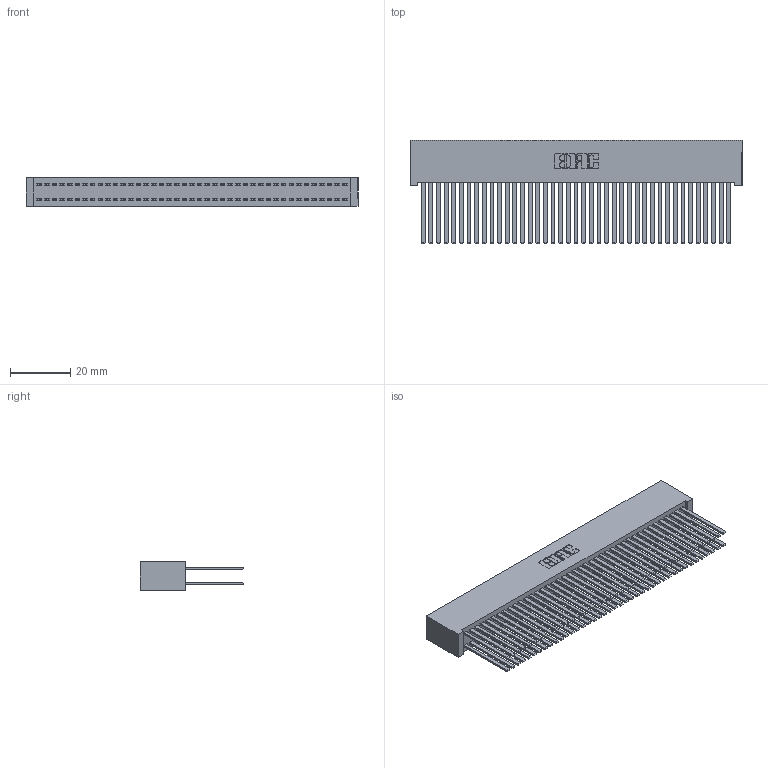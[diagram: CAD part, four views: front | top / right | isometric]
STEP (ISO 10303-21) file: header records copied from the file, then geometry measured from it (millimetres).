
FILE_DESCRIPTION (( 'STEP AP203' ), '1' );
FILE_NAME ('342-082-544-201.STEP', '2019-10-04T12:13:11', ( '' ), ( '' ), 'SwSTEP 2.0', 'SolidWorks 2016', '' );
FILE_SCHEMA (( 'CONFIG_CONTROL_DESIGN' ));
Length unit declared in the file: inch
Products named in the file (3): 342-082-544-201; 342 Part_Lugless; 345-292-001_345-293-144
Assembly tree (83 placements, depth 2):
  342-082-544-201
    342 Part_Lugless
    345-292-001_345-293-144  x82
Bounding box: 110.39 x 34.3 x 9.4 mm (x, y, z)
Volume: 11502.6 mm3; surface area: 22328.4 mm2
Topology: 83 solids, 83 shells, 3874 faces, 11509 edges, 7562 vertices
Faces by surface type: plane 2686, cylinder 1188
Entity records: 25913 total; most frequent: CARTESIAN_POINT 4290, ORIENTED_EDGE 4226, DIRECTION 3657, EDGE_CURVE 2113, LINE 1997, VECTOR 1997, VERTEX_POINT 1406, AXIS2_PLACEMENT_3D 830
